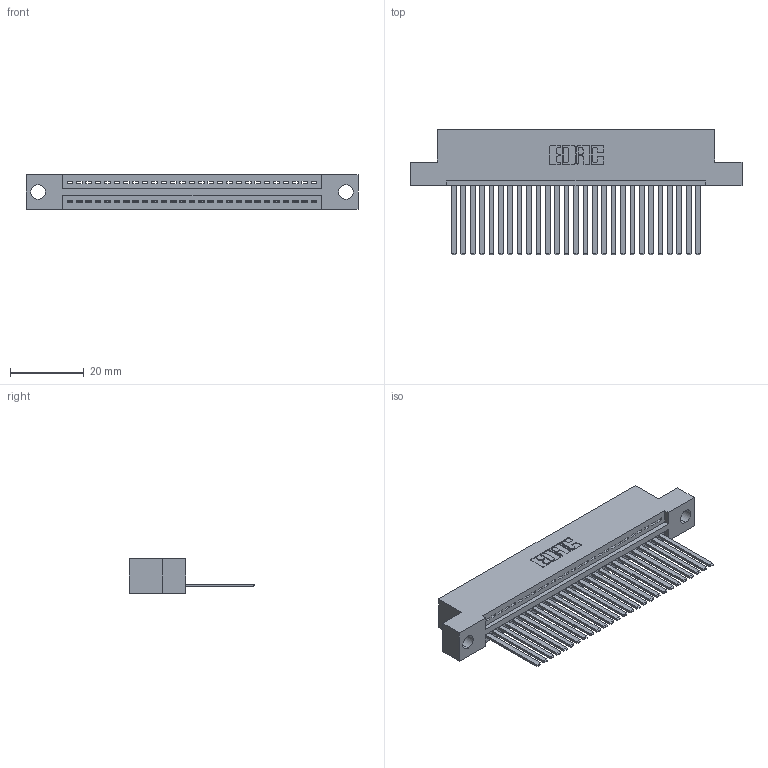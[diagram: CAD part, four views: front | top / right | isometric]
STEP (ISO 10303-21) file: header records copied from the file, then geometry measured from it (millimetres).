
FILE_DESCRIPTION (( 'STEP AP203' ), '1' );
FILE_NAME ('345-027-544-104.STEP', '2021-05-26T14:33:46', ( '' ), ( '' ), 'SwSTEP 2.0', 'SolidWorks 2020', '' );
FILE_SCHEMA (( 'CONFIG_CONTROL_DESIGN' ));
Length unit declared in the file: inch
Products named in the file (3): 345-292-001_345-293-144; 345-027-544-104; 345 Part_Flush Mounting Lugs - 0.156 Dia-TI
Assembly tree (28 placements, depth 2):
  345-027-544-104
    345 Part_Flush Mounting Lugs - 0.156 Dia-TI
    345-292-001_345-293-144  x27
Bounding box: 89.79 x 33.96 x 9.4 mm (x, y, z)
Volume: 8612.1 mm3; surface area: 12022.1 mm2
Topology: 28 solids, 28 shells, 1544 faces, 4643 edges, 3058 vertices
Faces by surface type: plane 1066, cylinder 478
Entity records: 22575 total; most frequent: CARTESIAN_POINT 3919, ORIENTED_EDGE 3878, DIRECTION 3441, EDGE_CURVE 1939, LINE 1703, VECTOR 1703, VERTEX_POINT 1290, AXIS2_PLACEMENT_3D 869
